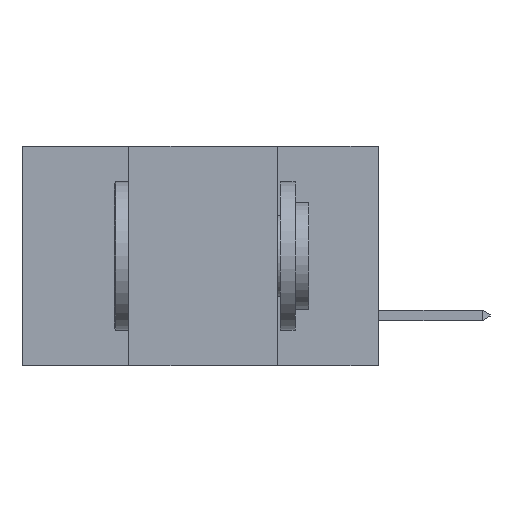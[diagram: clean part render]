
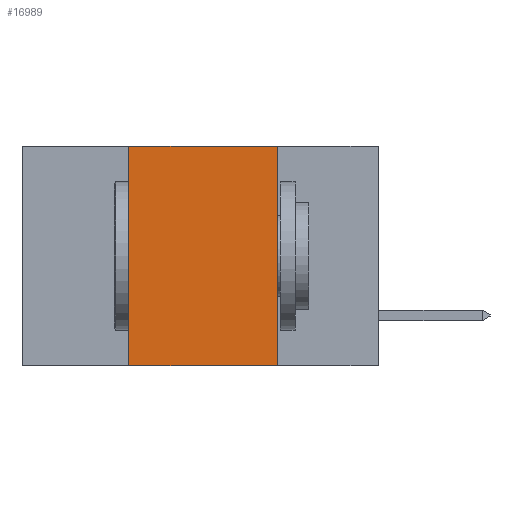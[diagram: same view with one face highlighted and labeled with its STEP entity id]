
A CAD part, left-side view. The second image highlights one B-rep face of the part: STEP entity #16989.
In plain terms, the highlighted planar face has unit normal (-1, 0, 0).
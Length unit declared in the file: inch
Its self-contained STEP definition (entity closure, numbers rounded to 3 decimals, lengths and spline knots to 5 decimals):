
#498 = EDGE_CURVE ( 'NONE', #1036, #9438, #16464, .T. ) ;
#821 = ORIENTED_EDGE ( 'NONE', *, *, #498, .T. ) ;
#1036 = VERTEX_POINT ( 'NONE', #9994 ) ;
#1755 = VERTEX_POINT ( 'NONE', #16413 ) ;
#1911 = EDGE_CURVE ( 'NONE', #1036, #1755, #9228, .T. ) ;
#2775 = PLANE ( 'NONE',  #6526 ) ;
#2899 = VERTEX_POINT ( 'NONE', #19988 ) ;
#4820 = CARTESIAN_POINT ( 'NONE',  ( 0., 0.6, 0. ) ) ;
#6034 = EDGE_CURVE ( 'NONE', #1755, #2899, #9669, .T. ) ;
#6526 = AXIS2_PLACEMENT_3D ( 'NONE', #4820, #8847, #22942 ) ;
#6830 = DIRECTION ( 'NONE',  ( 0., 0., -1. ) ) ;
#6951 = VECTOR ( 'NONE', #6830, 39.37008 ) ;
#7392 = EDGE_CURVE ( 'NONE', #2899, #9438, #22988, .T. ) ;
#8847 = DIRECTION ( 'NONE',  ( 1., 0., 0. ) ) ;
#9228 = LINE ( 'NONE', #13837, #24635 ) ;
#9360 = ORIENTED_EDGE ( 'NONE', *, *, #7392, .F. ) ;
#9438 = VERTEX_POINT ( 'NONE', #25484 ) ;
#9669 = LINE ( 'NONE', #22366, #14452 ) ;
#9994 = CARTESIAN_POINT ( 'NONE',  ( 0., 0.42, -0.37 ) ) ;
#10679 = ORIENTED_EDGE ( 'NONE', *, *, #1911, .F. ) ;
#11059 = EDGE_LOOP ( 'NONE', ( #9360, #18255, #10679, #821 ) ) ;
#13514 = DIRECTION ( 'NONE',  ( 0., 0., 1. ) ) ;
#13837 = CARTESIAN_POINT ( 'NONE',  ( 0., 0.42, -0.37 ) ) ;
#14452 = VECTOR ( 'NONE', #18701, 39.37008 ) ;
#14599 = VECTOR ( 'NONE', #24141, 39.37008 ) ;
#16413 = CARTESIAN_POINT ( 'NONE',  ( 0., 0.42, 0. ) ) ;
#16464 = LINE ( 'NONE', #20782, #14599 ) ;
#16989 = ADVANCED_FACE ( 'NONE', ( #20984 ), #2775, .F. ) ;
#18255 = ORIENTED_EDGE ( 'NONE', *, *, #6034, .F. ) ;
#18701 = DIRECTION ( 'NONE',  ( 0., -1., 0. ) ) ;
#19988 = CARTESIAN_POINT ( 'NONE',  ( 0., 0.17, 0. ) ) ;
#20782 = CARTESIAN_POINT ( 'NONE',  ( 0., 0.6, -0.37 ) ) ;
#20919 = CARTESIAN_POINT ( 'NONE',  ( 0., 0.17, -0.37 ) ) ;
#20984 = FACE_OUTER_BOUND ( 'NONE', #11059, .T. ) ;
#22366 = CARTESIAN_POINT ( 'NONE',  ( 0., 0.6, 0. ) ) ;
#22942 = DIRECTION ( 'NONE',  ( 0., 0., -1. ) ) ;
#22988 = LINE ( 'NONE', #20919, #6951 ) ;
#24141 = DIRECTION ( 'NONE',  ( 0., -1., 0. ) ) ;
#24635 = VECTOR ( 'NONE', #13514, 39.37008 ) ;
#25484 = CARTESIAN_POINT ( 'NONE',  ( 0., 0.17, -0.37 ) ) ;
